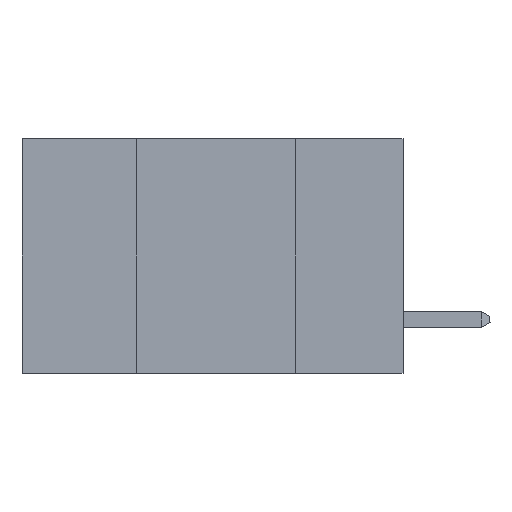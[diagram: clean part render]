
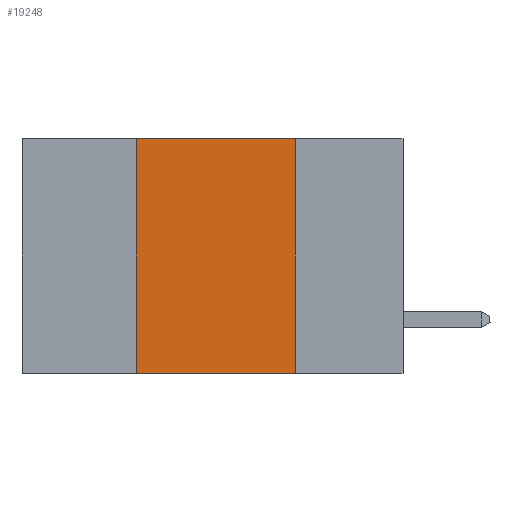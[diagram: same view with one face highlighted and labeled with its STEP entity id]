
A CAD part, left-side view. The second image highlights one B-rep face of the part: STEP entity #19248.
In plain terms, the highlighted planar face has unit normal (-1, 0, 0).
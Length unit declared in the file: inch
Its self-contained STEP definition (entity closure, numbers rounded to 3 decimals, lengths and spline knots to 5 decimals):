
#443 = AXIS2_PLACEMENT_3D ( 'NONE', #9254, #29732, #12232 ) ;
#1549 = CARTESIAN_POINT ( 'NONE',  ( 0., 0.6, 0. ) ) ;
#4308 = VECTOR ( 'NONE', #7928, 39.37008 ) ;
#4956 = CARTESIAN_POINT ( 'NONE',  ( 0., 0.42, 0. ) ) ;
#6209 = VERTEX_POINT ( 'NONE', #24354 ) ;
#6913 = EDGE_CURVE ( 'NONE', #33214, #6209, #20585, .T. ) ;
#7162 = DIRECTION ( 'NONE',  ( 0., -1., 0. ) ) ;
#7670 = EDGE_CURVE ( 'NONE', #33616, #12590, #10068, .T. ) ;
#7928 = DIRECTION ( 'NONE',  ( 0., 0., 1. ) ) ;
#9254 = CARTESIAN_POINT ( 'NONE',  ( 0., 0.6, 0. ) ) ;
#10068 = LINE ( 'NONE', #1549, #16933 ) ;
#10422 = CARTESIAN_POINT ( 'NONE',  ( 0., 0.42, 0. ) ) ;
#10924 = ORIENTED_EDGE ( 'NONE', *, *, #6913, .T. ) ;
#11254 = LINE ( 'NONE', #4956, #4308 ) ;
#12232 = DIRECTION ( 'NONE',  ( 0., 0., -1. ) ) ;
#12590 = VERTEX_POINT ( 'NONE', #35602 ) ;
#15203 = ORIENTED_EDGE ( 'NONE', *, *, #24260, .F. ) ;
#16933 = VECTOR ( 'NONE', #25035, 39.37008 ) ;
#18396 = LINE ( 'NONE', #23475, #33039 ) ;
#19248 = ADVANCED_FACE ( 'NONE', ( #22426 ), #35457, .F. ) ;
#20585 = LINE ( 'NONE', #36325, #28395 ) ;
#21687 = EDGE_LOOP ( 'NONE', ( #15203, #22311, #29413, #10924 ) ) ;
#22311 = ORIENTED_EDGE ( 'NONE', *, *, #7670, .F. ) ;
#22426 = FACE_OUTER_BOUND ( 'NONE', #21687, .T. ) ;
#23475 = CARTESIAN_POINT ( 'NONE',  ( 0., 0.17, 0. ) ) ;
#24260 = EDGE_CURVE ( 'NONE', #12590, #6209, #18396, .T. ) ;
#24354 = CARTESIAN_POINT ( 'NONE',  ( 0., 0.17, -0.37 ) ) ;
#25035 = DIRECTION ( 'NONE',  ( 0., -1., 0. ) ) ;
#26418 = DIRECTION ( 'NONE',  ( 0., 0., -1. ) ) ;
#28395 = VECTOR ( 'NONE', #7162, 39.37008 ) ;
#29116 = CARTESIAN_POINT ( 'NONE',  ( 0., 0.42, -0.37 ) ) ;
#29413 = ORIENTED_EDGE ( 'NONE', *, *, #36017, .F. ) ;
#29732 = DIRECTION ( 'NONE',  ( 1., 0., 0. ) ) ;
#33039 = VECTOR ( 'NONE', #26418, 39.37008 ) ;
#33214 = VERTEX_POINT ( 'NONE', #29116 ) ;
#33616 = VERTEX_POINT ( 'NONE', #10422 ) ;
#35457 = PLANE ( 'NONE',  #443 ) ;
#35602 = CARTESIAN_POINT ( 'NONE',  ( 0., 0.17, 0. ) ) ;
#36017 = EDGE_CURVE ( 'NONE', #33214, #33616, #11254, .T. ) ;
#36325 = CARTESIAN_POINT ( 'NONE',  ( 0., 0.6, -0.37 ) ) ;
